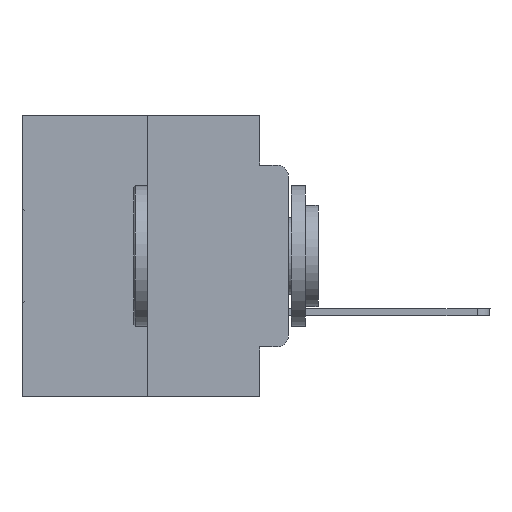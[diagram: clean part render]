
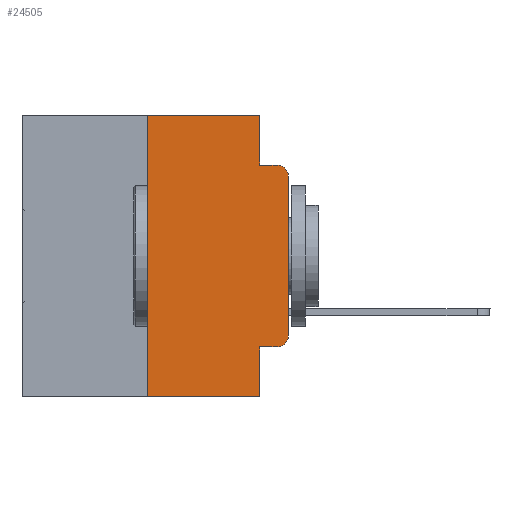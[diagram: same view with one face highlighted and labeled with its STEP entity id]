
A CAD part, left-side view. The second image highlights one B-rep face of the part: STEP entity #24505.
In plain terms, the highlighted planar face has unit normal (-1, 0, 0).
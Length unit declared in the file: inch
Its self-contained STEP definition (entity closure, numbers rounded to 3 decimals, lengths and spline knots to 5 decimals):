
#413 = CARTESIAN_POINT ( 'NONE',  ( 0., 0.02, -0.1085 ) ) ;
#952 = EDGE_CURVE ( 'NONE', #26053, #7506, #8108, .T. ) ;
#1160 = VECTOR ( 'NONE', #6964, 39.37008 ) ;
#1492 = FACE_OUTER_BOUND ( 'NONE', #14995, .T. ) ;
#1867 = CARTESIAN_POINT ( 'NONE',  ( 0., 0.02, -0.4115 ) ) ;
#2690 = DIRECTION ( 'NONE',  ( 0., 0., -1. ) ) ;
#3256 = LINE ( 'NONE', #23544, #15281 ) ;
#3299 = VECTOR ( 'NONE', #5347, 39.37008 ) ;
#3759 = EDGE_CURVE ( 'NONE', #5787, #8288, #22645, .T. ) ;
#4018 = CARTESIAN_POINT ( 'NONE',  ( 0., 0., -0.1085 ) ) ;
#4111 = LINE ( 'NONE', #27584, #22205 ) ;
#4929 = ORIENTED_EDGE ( 'NONE', *, *, #952, .T. ) ;
#5347 = DIRECTION ( 'NONE',  ( 0., 0., 1. ) ) ;
#5394 = ORIENTED_EDGE ( 'NONE', *, *, #3759, .F. ) ;
#5481 = AXIS2_PLACEMENT_3D ( 'NONE', #13682, #28230, #28440 ) ;
#5531 = DIRECTION ( 'NONE',  ( 0., -1., 0. ) ) ;
#5562 = CARTESIAN_POINT ( 'NONE',  ( 0., 0.02, -0.0885 ) ) ;
#5787 = VERTEX_POINT ( 'NONE', #25769 ) ;
#6964 = DIRECTION ( 'NONE',  ( 0., -1., 0. ) ) ;
#7340 = CARTESIAN_POINT ( 'NONE',  ( 0., 0.051, 0. ) ) ;
#7506 = VERTEX_POINT ( 'NONE', #1867 ) ;
#7732 = VECTOR ( 'NONE', #19345, 39.37008 ) ;
#8108 = LINE ( 'NONE', #11451, #20156 ) ;
#8153 = ORIENTED_EDGE ( 'NONE', *, *, #16217, .T. ) ;
#8288 = VERTEX_POINT ( 'NONE', #5562 ) ;
#8427 = VECTOR ( 'NONE', #20506, 39.37008 ) ;
#8930 = VERTEX_POINT ( 'NONE', #4018 ) ;
#9336 = LINE ( 'NONE', #10288, #3299 ) ;
#9622 = LINE ( 'NONE', #7340, #7732 ) ;
#9905 = EDGE_CURVE ( 'NONE', #26053, #22674, #9622, .T. ) ;
#10288 = CARTESIAN_POINT ( 'NONE',  ( 0., 0., 0. ) ) ;
#11451 = CARTESIAN_POINT ( 'NONE',  ( 0., 0.051, -0.4115 ) ) ;
#12010 = VECTOR ( 'NONE', #5531, 39.37008 ) ;
#12050 = CARTESIAN_POINT ( 'NONE',  ( 0., 0.051, 0. ) ) ;
#12166 = EDGE_CURVE ( 'NONE', #28866, #23122, #30482, .T. ) ;
#13300 = VERTEX_POINT ( 'NONE', #30458 ) ;
#13606 = CARTESIAN_POINT ( 'NONE',  ( 0., 0.25, 0. ) ) ;
#13682 = CARTESIAN_POINT ( 'NONE',  ( 0., 0.473, 0. ) ) ;
#13837 = CARTESIAN_POINT ( 'NONE',  ( 0., 0.02, -0.3915 ) ) ;
#14688 = ORIENTED_EDGE ( 'NONE', *, *, #25267, .T. ) ;
#14872 = EDGE_CURVE ( 'NONE', #7506, #13300, #27227, .T. ) ;
#14995 = EDGE_LOOP ( 'NONE', ( #14688, #8153, #5394, #24732, #30698, #18258, #18110, #16943, #4929, #20376 ) ) ;
#15281 = VECTOR ( 'NONE', #30706, 39.37008 ) ;
#16119 = PLANE ( 'NONE',  #5481 ) ;
#16217 = EDGE_CURVE ( 'NONE', #8930, #8288, #25758, .T. ) ;
#16492 = DIRECTION ( 'NONE',  ( 0., 0., -1. ) ) ;
#16943 = ORIENTED_EDGE ( 'NONE', *, *, #9905, .F. ) ;
#17620 = CARTESIAN_POINT ( 'NONE',  ( 0., 0.473, 0. ) ) ;
#18110 = ORIENTED_EDGE ( 'NONE', *, *, #22997, .T. ) ;
#18258 = ORIENTED_EDGE ( 'NONE', *, *, #24404, .F. ) ;
#18819 = DIRECTION ( 'NONE',  ( -1., 0., 0. ) ) ;
#18857 = CARTESIAN_POINT ( 'NONE',  ( 0., 0.051, -0.0885 ) ) ;
#19345 = DIRECTION ( 'NONE',  ( 0., 0., -1. ) ) ;
#19736 = DIRECTION ( 'NONE',  ( -1., 0., 0. ) ) ;
#20067 = CARTESIAN_POINT ( 'NONE',  ( 0., 0.051, -0.5 ) ) ;
#20156 = VECTOR ( 'NONE', #28388, 39.37008 ) ;
#20376 = ORIENTED_EDGE ( 'NONE', *, *, #14872, .T. ) ;
#20506 = DIRECTION ( 'NONE',  ( 0., 0., -1. ) ) ;
#20699 = VERTEX_POINT ( 'NONE', #28512 ) ;
#22205 = VECTOR ( 'NONE', #22900, 39.37008 ) ;
#22645 = LINE ( 'NONE', #18857, #1160 ) ;
#22674 = VERTEX_POINT ( 'NONE', #20067 ) ;
#22900 = DIRECTION ( 'NONE',  ( 0., 0., 1. ) ) ;
#22903 = AXIS2_PLACEMENT_3D ( 'NONE', #413, #19736, #2690 ) ;
#22997 = EDGE_CURVE ( 'NONE', #20699, #22674, #3256, .T. ) ;
#23102 = AXIS2_PLACEMENT_3D ( 'NONE', #13837, #18819, #16492 ) ;
#23122 = VERTEX_POINT ( 'NONE', #12050 ) ;
#23544 = CARTESIAN_POINT ( 'NONE',  ( 0., 0.473, -0.5 ) ) ;
#24404 = EDGE_CURVE ( 'NONE', #20699, #28866, #4111, .T. ) ;
#24505 = ADVANCED_FACE ( 'NONE', ( #1492 ), #16119, .F. ) ;
#24732 = ORIENTED_EDGE ( 'NONE', *, *, #31125, .F. ) ;
#25267 = EDGE_CURVE ( 'NONE', #13300, #8930, #9336, .T. ) ;
#25385 = CARTESIAN_POINT ( 'NONE',  ( 0., 0.051, 0. ) ) ;
#25758 = CIRCLE ( 'NONE', #22903, 0.02 ) ;
#25769 = CARTESIAN_POINT ( 'NONE',  ( 0., 0.051, -0.0885 ) ) ;
#26053 = VERTEX_POINT ( 'NONE', #29427 ) ;
#26506 = LINE ( 'NONE', #25385, #8427 ) ;
#27227 = CIRCLE ( 'NONE', #23102, 0.02 ) ;
#27584 = CARTESIAN_POINT ( 'NONE',  ( 0., 0.25, 0. ) ) ;
#28230 = DIRECTION ( 'NONE',  ( 1., 0., 0. ) ) ;
#28388 = DIRECTION ( 'NONE',  ( 0., -1., 0. ) ) ;
#28440 = DIRECTION ( 'NONE',  ( 0., 0., -1. ) ) ;
#28512 = CARTESIAN_POINT ( 'NONE',  ( 0., 0.25, -0.5 ) ) ;
#28866 = VERTEX_POINT ( 'NONE', #13606 ) ;
#29427 = CARTESIAN_POINT ( 'NONE',  ( 0., 0.051, -0.4115 ) ) ;
#30458 = CARTESIAN_POINT ( 'NONE',  ( 0., 0., -0.3915 ) ) ;
#30482 = LINE ( 'NONE', #17620, #12010 ) ;
#30698 = ORIENTED_EDGE ( 'NONE', *, *, #12166, .F. ) ;
#30706 = DIRECTION ( 'NONE',  ( 0., -1., 0. ) ) ;
#31125 = EDGE_CURVE ( 'NONE', #23122, #5787, #26506, .T. ) ;
